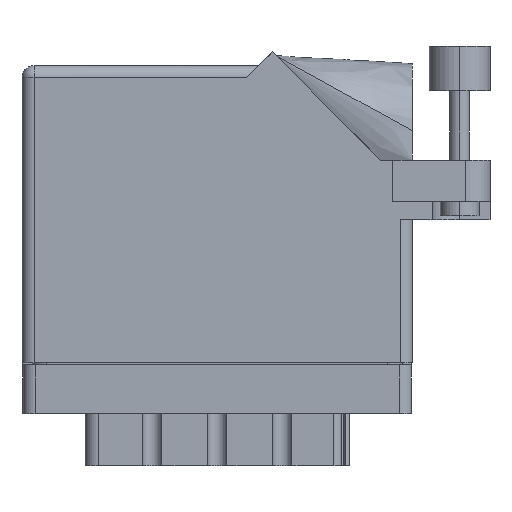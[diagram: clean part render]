
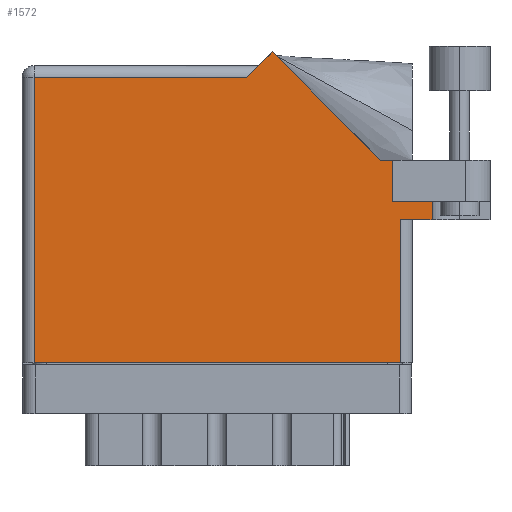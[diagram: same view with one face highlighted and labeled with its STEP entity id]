
A CAD part, front view. The second image highlights one B-rep face of the part: STEP entity #1572.
In plain terms, the highlighted face is planar.
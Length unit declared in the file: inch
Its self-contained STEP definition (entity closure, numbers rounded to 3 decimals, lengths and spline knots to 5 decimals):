
#861 = ORIENTED_EDGE ( 'NONE', *, *, #17793, .T. ) ;
#978 = DIRECTION ( 'NONE',  ( 1., 0., 0. ) ) ;
#1572 = ADVANCED_FACE ( 'NONE', ( #3701 ), #28553, .F. ) ;
#1717 = EDGE_CURVE ( 'NONE', #39837, #28937, #14788, .T. ) ;
#2856 = AXIS2_PLACEMENT_3D ( 'NONE', #15788, #22215, #34707 ) ;
#2948 = EDGE_CURVE ( 'NONE', #40883, #37511, #17697, .T. ) ;
#3701 = FACE_OUTER_BOUND ( 'NONE', #26009, .T. ) ;
#3734 = VERTEX_POINT ( 'NONE', #19934 ) ;
#3856 = ORIENTED_EDGE ( 'NONE', *, *, #18474, .T. ) ;
#4118 = CARTESIAN_POINT ( 'NONE',  ( 1.28771, 1.60071, 0. ) ) ;
#4292 = VERTEX_POINT ( 'NONE', #4118 ) ;
#4347 = DIRECTION ( 'NONE',  ( -0.707, -0.707, 0. ) ) ;
#4707 = CARTESIAN_POINT ( 'NONE',  ( 2.41, 1.044, 0. ) ) ;
#4945 = EDGE_CURVE ( 'NONE', #4292, #7993, #14506, .T. ) ;
#5773 = DIRECTION ( 'NONE',  ( -0.707, 0.707, 0. ) ) ;
#6582 = CARTESIAN_POINT ( 'NONE',  ( 1.91, 0.831, 0. ) ) ;
#7555 = ORIENTED_EDGE ( 'NONE', *, *, #2948, .F. ) ;
#7676 = LINE ( 'NONE', #11138, #15810 ) ;
#7993 = VERTEX_POINT ( 'NONE', #28799 ) ;
#8221 = EDGE_CURVE ( 'NONE', #23976, #36205, #16077, .T. ) ;
#8349 = CARTESIAN_POINT ( 'NONE',  ( 2.1115, 0.831, 0. ) ) ;
#8682 = EDGE_CURVE ( 'NONE', #37511, #36205, #7676, .T. ) ;
#10757 = DIRECTION ( 'NONE',  ( -1., 0., 0. ) ) ;
#11138 = CARTESIAN_POINT ( 'NONE',  ( 2.1115, 1.16177, 0. ) ) ;
#12645 = ORIENTED_EDGE ( 'NONE', *, *, #26372, .T. ) ;
#12964 = DIRECTION ( 'NONE',  ( 1., 0., 0. ) ) ;
#14135 = ORIENTED_EDGE ( 'NONE', *, *, #15406, .T. ) ;
#14506 = LINE ( 'NONE', #26271, #26533 ) ;
#14788 = LINE ( 'NONE', #35536, #24806 ) ;
#15406 = EDGE_CURVE ( 'NONE', #15556, #22850, #28629, .T. ) ;
#15556 = VERTEX_POINT ( 'NONE', #34630 ) ;
#15788 = CARTESIAN_POINT ( 'NONE',  ( 0., 1.53, 0. ) ) ;
#15810 = VECTOR ( 'NONE', #27184, 39.37008 ) ;
#15966 = CARTESIAN_POINT ( 'NONE',  ( 2.01, 0.737, 0. ) ) ;
#16077 = LINE ( 'NONE', #15966, #23538 ) ;
#16218 = VECTOR ( 'NONE', #978, 39.37008 ) ;
#16737 = CARTESIAN_POINT ( 'NONE',  ( 1.91, 0.831, 0. ) ) ;
#17697 = LINE ( 'NONE', #16737, #16218 ) ;
#17793 = EDGE_CURVE ( 'NONE', #40883, #15556, #27433, .T. ) ;
#17817 = LINE ( 'NONE', #28734, #30361 ) ;
#18037 = CARTESIAN_POINT ( 'NONE',  ( 2.1115, 0.737, 0. ) ) ;
#18474 = EDGE_CURVE ( 'NONE', #22850, #4292, #17817, .T. ) ;
#18528 = ORIENTED_EDGE ( 'NONE', *, *, #4945, .T. ) ;
#19039 = CARTESIAN_POINT ( 'NONE',  ( 1.84442, 1.044, 0. ) ) ;
#19934 = CARTESIAN_POINT ( 'NONE',  ( 1.948, 0., 0. ) ) ;
#20025 = CARTESIAN_POINT ( 'NONE',  ( 0.062, 0., 0. ) ) ;
#20376 = VECTOR ( 'NONE', #28369, 39.37008 ) ;
#20595 = CARTESIAN_POINT ( 'NONE',  ( 0.062, 1.468, 0. ) ) ;
#20597 = VECTOR ( 'NONE', #10757, 39.37008 ) ;
#20709 = DIRECTION ( 'NONE',  ( 0., 1., 0. ) ) ;
#20736 = EDGE_CURVE ( 'NONE', #28937, #3734, #22219, .T. ) ;
#22076 = VECTOR ( 'NONE', #31250, 39.37008 ) ;
#22215 = DIRECTION ( 'NONE',  ( 0., 0., -1. ) ) ;
#22219 = LINE ( 'NONE', #35737, #27206 ) ;
#22850 = VERTEX_POINT ( 'NONE', #19039 ) ;
#23538 = VECTOR ( 'NONE', #12964, 39.37008 ) ;
#23976 = VERTEX_POINT ( 'NONE', #24822 ) ;
#24753 = ORIENTED_EDGE ( 'NONE', *, *, #20736, .T. ) ;
#24806 = VECTOR ( 'NONE', #32412, 39.37008 ) ;
#24822 = CARTESIAN_POINT ( 'NONE',  ( 1.948, 0.737, 0. ) ) ;
#25426 = LINE ( 'NONE', #39874, #36467 ) ;
#26009 = EDGE_LOOP ( 'NONE', ( #24753, #38374, #38926, #36031, #7555, #861, #14135, #3856, #18528, #12645, #27988 ) ) ;
#26174 = DIRECTION ( 'NONE',  ( 1., 0., 0. ) ) ;
#26271 = CARTESIAN_POINT ( 'NONE',  ( 1.217, 1.53, 0. ) ) ;
#26372 = EDGE_CURVE ( 'NONE', #7993, #39837, #29157, .T. ) ;
#26533 = VECTOR ( 'NONE', #4347, 39.37008 ) ;
#26786 = CARTESIAN_POINT ( 'NONE',  ( 0., 1.468, 0. ) ) ;
#27184 = DIRECTION ( 'NONE',  ( 0., -1., 0. ) ) ;
#27206 = VECTOR ( 'NONE', #26174, 39.37008 ) ;
#27433 = LINE ( 'NONE', #41053, #20376 ) ;
#27988 = ORIENTED_EDGE ( 'NONE', *, *, #1717, .T. ) ;
#28369 = DIRECTION ( 'NONE',  ( 0., 1., 0. ) ) ;
#28553 = PLANE ( 'NONE',  #2856 ) ;
#28629 = LINE ( 'NONE', #4707, #22076 ) ;
#28734 = CARTESIAN_POINT ( 'NONE',  ( 1.84442, 1.044, 0. ) ) ;
#28799 = CARTESIAN_POINT ( 'NONE',  ( 1.155, 1.468, 0. ) ) ;
#28937 = VERTEX_POINT ( 'NONE', #20025 ) ;
#29054 = EDGE_CURVE ( 'NONE', #3734, #23976, #25426, .T. ) ;
#29157 = LINE ( 'NONE', #26786, #20597 ) ;
#30361 = VECTOR ( 'NONE', #5773, 39.37008 ) ;
#31250 = DIRECTION ( 'NONE',  ( -1., 0., 0. ) ) ;
#32412 = DIRECTION ( 'NONE',  ( 0., -1., 0. ) ) ;
#34630 = CARTESIAN_POINT ( 'NONE',  ( 1.91, 1.044, 0. ) ) ;
#34707 = DIRECTION ( 'NONE',  ( -1., 0., 0. ) ) ;
#35536 = CARTESIAN_POINT ( 'NONE',  ( 0.062, 0., 0. ) ) ;
#35737 = CARTESIAN_POINT ( 'NONE',  ( 0., 0., 0. ) ) ;
#36031 = ORIENTED_EDGE ( 'NONE', *, *, #8682, .F. ) ;
#36205 = VERTEX_POINT ( 'NONE', #18037 ) ;
#36467 = VECTOR ( 'NONE', #20709, 39.37008 ) ;
#37511 = VERTEX_POINT ( 'NONE', #8349 ) ;
#38374 = ORIENTED_EDGE ( 'NONE', *, *, #29054, .T. ) ;
#38926 = ORIENTED_EDGE ( 'NONE', *, *, #8221, .T. ) ;
#39837 = VERTEX_POINT ( 'NONE', #20595 ) ;
#39874 = CARTESIAN_POINT ( 'NONE',  ( 1.948, 0.737, 0. ) ) ;
#40883 = VERTEX_POINT ( 'NONE', #6582 ) ;
#41053 = CARTESIAN_POINT ( 'NONE',  ( 1.91, 0.831, 0. ) ) ;
